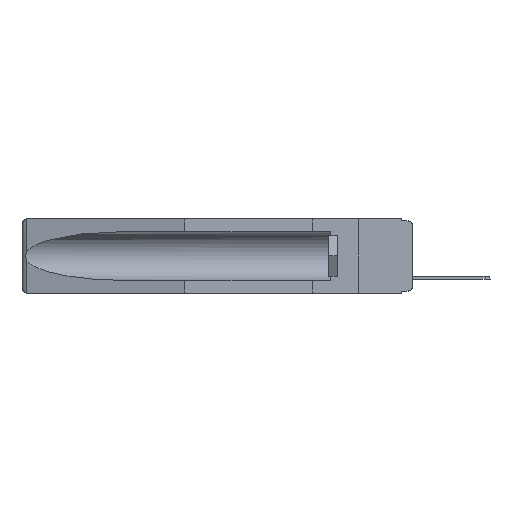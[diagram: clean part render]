
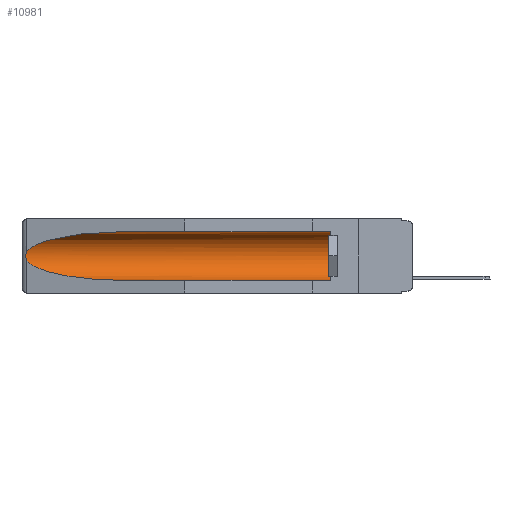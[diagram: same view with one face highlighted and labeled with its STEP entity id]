
A CAD part, left-side view. The second image highlights one B-rep face of the part: STEP entity #10981.
In plain terms, the highlighted cylindrical face has radius 2.857 mm (diameter 5.715 mm), a partial arc.
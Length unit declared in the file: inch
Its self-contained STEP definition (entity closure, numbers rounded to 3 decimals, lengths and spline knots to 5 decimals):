
#75 = CARTESIAN_POINT ( 'NONE',  ( 0.26537, 1.52718, -0.19328 ) ) ;
#367 = LINE ( 'NONE', #16639, #10663 ) ;
#375 = AXIS2_PLACEMENT_3D ( 'NONE', #4789, #10604, #7640 ) ;
#387 = CARTESIAN_POINT ( 'NONE',  ( 0.21114, 1.30732, -0.284 ) ) ;
#1628 = CARTESIAN_POINT ( 'NONE',  ( 0.155, 0.126, -0.1715 ) ) ;
#3639 = CARTESIAN_POINT ( 'NONE',  ( 0.155, -0.30754, -0.059 ) ) ;
#3857 = VECTOR ( 'NONE', #15077, 39.37008 ) ;
#3931 = VERTEX_POINT ( 'NONE', #13077 ) ;
#4371 = CARTESIAN_POINT ( 'NONE',  ( 0.26537, 1.52718, -0.14972 ) ) ;
#4494 = CARTESIAN_POINT ( 'NONE',  ( 0.2675, 1.53308, -0.17534 ) ) ;
#4555 = CARTESIAN_POINT ( 'NONE',  ( 0.26597, 1.5296, -0.19026 ) ) ;
#4789 = CARTESIAN_POINT ( 'NONE',  ( 0.155, -0.30754, -0.1715 ) ) ;
#4929 = EDGE_CURVE ( 'NONE', #3931, #6388, #16596, .T. ) ;
#5773 = DIRECTION ( 'NONE',  ( 0., 0., 1. ) ) ;
#5840 = DIRECTION ( 'NONE',  ( 0., -1., 0. ) ) ;
#6109 = CARTESIAN_POINT ( 'NONE',  ( 0.26537, 1.52718, -0.19328 ) ) ;
#6388 = VERTEX_POINT ( 'NONE', #75 ) ;
#6554 = LINE ( 'NONE', #3639, #3857 ) ;
#6929 = ORIENTED_EDGE ( 'NONE', *, *, #4929, .T. ) ;
#7161 = EDGE_CURVE ( 'NONE', #17606, #16398, #6554, .T. ) ;
#7342 = CYLINDRICAL_SURFACE ( 'NONE', #375, 0.1125 ) ;
#7559 = CARTESIAN_POINT ( 'NONE',  ( 0.155, 1.07973, -0.284 ) ) ;
#7640 = DIRECTION ( 'NONE',  ( 0., 0., 1. ) ) ;
#8305 = AXIS2_PLACEMENT_3D ( 'NONE', #1628, #5840, #5773 ) ;
#8333 = CARTESIAN_POINT ( 'NONE',  ( 0.26537, 1.52718, -0.14972 ) ) ;
#8460 = EDGE_CURVE ( 'NONE', #16398, #3931, #15450, .T. ) ;
#8712 = CARTESIAN_POINT ( 'NONE',  ( 0.2673, 1.53269, -0.17917 ) ) ;
#9562 = CARTESIAN_POINT ( 'NONE',  ( 0.155, 0.126, -0.284 ) ) ;
#9730 = ORIENTED_EDGE ( 'NONE', *, *, #7161, .T. ) ;
#9998 = CARTESIAN_POINT ( 'NONE',  ( 0.26597, 1.52961, -0.15275 ) ) ;
#10221 = CARTESIAN_POINT ( 'NONE',  ( 0.155, 1.07973, -0.059 ) ) ;
#10243 = ORIENTED_EDGE ( 'NONE', *, *, #18341, .T. ) ;
#10604 = DIRECTION ( 'NONE',  ( 0., 1., 0. ) ) ;
#10663 = VECTOR ( 'NONE', #11008, 39.37008 ) ;
#10681 = VERTEX_POINT ( 'NONE', #9562 ) ;
#10981 = ADVANCED_FACE ( 'NONE', ( #13142 ), #7342, .F. ) ;
#11008 = DIRECTION ( 'NONE',  ( 0., 1., 0. ) ) ;
#11044 = CARTESIAN_POINT ( 'NONE',  ( 0.21114, 1.30732, -0.059 ) ) ;
#11227 = CARTESIAN_POINT ( 'NONE',  ( 0.25451, 1.48313, -0.09465 ) ) ;
#11322 = CARTESIAN_POINT ( 'NONE',  ( 0.155, 1.07973, -0.284 ) ) ;
#11440 = EDGE_LOOP ( 'NONE', ( #18000, #6929, #10243, #11477, #17018, #9730 ) ) ;
#11477 = ORIENTED_EDGE ( 'NONE', *, *, #15952, .F. ) ;
#11619 = CARTESIAN_POINT ( 'NONE',  ( 0.2673, 1.5327, -0.16383 ) ) ;
#11682 = CARTESIAN_POINT ( 'NONE',  ( 0.26655, 1.53094, -0.18657 ) ) ;
#12104 =( BOUNDED_CURVE ( )  B_SPLINE_CURVE ( 3, ( #6109, #16119, #387, #7559 ),
 .UNSPECIFIED., .F., .T. ) 
 B_SPLINE_CURVE_WITH_KNOTS ( ( 4, 4 ),
 ( 0.1948, 1.5708 ),
 .UNSPECIFIED. ) 
 CURVE ( )  GEOMETRIC_REPRESENTATION_ITEM ( )  RATIONAL_B_SPLINE_CURVE ( ( 1., 0.848, 0.848, 1. ) ) 
 REPRESENTATION_ITEM ( '' )  );
#13052 = CARTESIAN_POINT ( 'NONE',  ( 0.2675, 1.53308, -0.16763 ) ) ;
#13077 = CARTESIAN_POINT ( 'NONE',  ( 0.26537, 1.52718, -0.14972 ) ) ;
#13142 = FACE_OUTER_BOUND ( 'NONE', #11440, .T. ) ;
#13361 = CARTESIAN_POINT ( 'NONE',  ( 0.155, 0.126, -0.059 ) ) ;
#14680 = CIRCLE ( 'NONE', #8305, 0.1125 ) ;
#15077 = DIRECTION ( 'NONE',  ( 0., 1., 0. ) ) ;
#15450 =( BOUNDED_CURVE ( )  B_SPLINE_CURVE ( 3, ( #16813, #11044, #11227, #8333 ),
 .UNSPECIFIED., .F., .F. ) 
 B_SPLINE_CURVE_WITH_KNOTS ( ( 4, 4 ),
 ( 4.71239, 6.08839 ),
 .UNSPECIFIED. ) 
 CURVE ( )  GEOMETRIC_REPRESENTATION_ITEM ( )  RATIONAL_B_SPLINE_CURVE ( ( 1., 0.848, 0.848, 1. ) ) 
 REPRESENTATION_ITEM ( '' )  );
#15511 = VERTEX_POINT ( 'NONE', #11322 ) ;
#15829 = CARTESIAN_POINT ( 'NONE',  ( 0.26654, 1.53092, -0.15636 ) ) ;
#15952 = EDGE_CURVE ( 'NONE', #10681, #15511, #367, .T. ) ;
#16119 = CARTESIAN_POINT ( 'NONE',  ( 0.25451, 1.48313, -0.24835 ) ) ;
#16398 = VERTEX_POINT ( 'NONE', #10221 ) ;
#16596 = B_SPLINE_CURVE_WITH_KNOTS ( 'NONE', 3,
 ( #4371, #9998, #15829, #11619, #13052, #4494, #8712, #11682, #4555, #17403 ),
 .UNSPECIFIED., .F., .F.,
 ( 4, 2, 2, 2, 4 ),
 ( 0., 0.00029, 0.00058, 0.00087, 0.00117 ),
 .UNSPECIFIED. ) ;
#16639 = CARTESIAN_POINT ( 'NONE',  ( 0.155, -0.30754, -0.284 ) ) ;
#16813 = CARTESIAN_POINT ( 'NONE',  ( 0.155, 1.07973, -0.059 ) ) ;
#16997 = EDGE_CURVE ( 'NONE', #10681, #17606, #14680, .T. ) ;
#17018 = ORIENTED_EDGE ( 'NONE', *, *, #16997, .T. ) ;
#17403 = CARTESIAN_POINT ( 'NONE',  ( 0.26537, 1.52718, -0.19328 ) ) ;
#17606 = VERTEX_POINT ( 'NONE', #13361 ) ;
#18000 = ORIENTED_EDGE ( 'NONE', *, *, #8460, .T. ) ;
#18341 = EDGE_CURVE ( 'NONE', #6388, #15511, #12104, .T. ) ;
